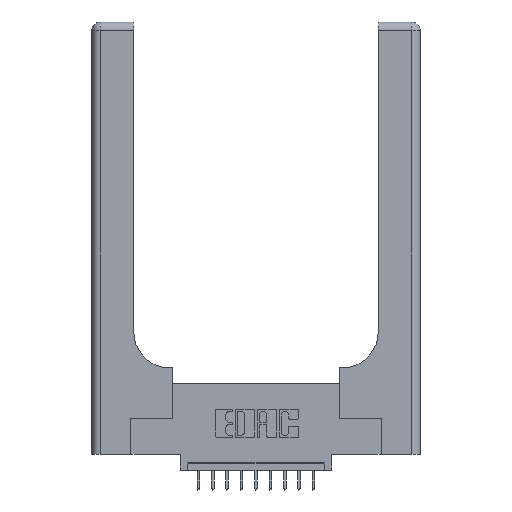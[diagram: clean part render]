
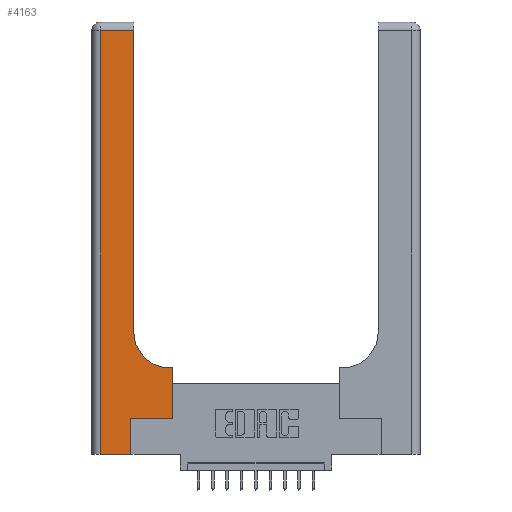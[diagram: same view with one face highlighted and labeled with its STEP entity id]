
A CAD part, top view. The second image highlights one B-rep face of the part: STEP entity #4163.
In plain terms, the highlighted planar face has unit normal (0, 0, 1).
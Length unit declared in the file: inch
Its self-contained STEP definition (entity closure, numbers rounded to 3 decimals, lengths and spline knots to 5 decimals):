
#88 = CARTESIAN_POINT ( 'NONE',  ( 0.5585, 0.6, 0.37 ) ) ;
#327 = VECTOR ( 'NONE', #10025, 39.37008 ) ;
#654 = ORIENTED_EDGE ( 'NONE', *, *, #2402, .T. ) ;
#759 = CARTESIAN_POINT ( 'NONE',  ( 0.5585, 0.25, 0.37 ) ) ;
#824 = CARTESIAN_POINT ( 'NONE',  ( 0.5415, 0.6, 0.37 ) ) ;
#992 = CARTESIAN_POINT ( 'NONE',  ( 0., 2.94, 0.37 ) ) ;
#1068 = VECTOR ( 'NONE', #10743, 39.37008 ) ;
#1175 = EDGE_CURVE ( 'NONE', #6383, #5302, #15178, .T. ) ;
#1339 = DIRECTION ( 'NONE',  ( 0., 1., 0. ) ) ;
#1602 = EDGE_LOOP ( 'NONE', ( #10691, #9504, #8121, #3384, #654, #14400, #3420, #8779, #9901 ) ) ;
#1735 = CARTESIAN_POINT ( 'NONE',  ( 0.269, 0., 0.37 ) ) ;
#2074 = EDGE_CURVE ( 'NONE', #12325, #16010, #11331, .T. ) ;
#2081 = CARTESIAN_POINT ( 'NONE',  ( 0.269, 0.25, 0.37 ) ) ;
#2402 = EDGE_CURVE ( 'NONE', #16010, #4941, #10570, .T. ) ;
#2519 = VECTOR ( 'NONE', #8267, 39.37008 ) ;
#2576 = EDGE_CURVE ( 'NONE', #12427, #7344, #16180, .T. ) ;
#3227 = CARTESIAN_POINT ( 'NONE',  ( 0.269, 0.25, 0.37 ) ) ;
#3384 = ORIENTED_EDGE ( 'NONE', *, *, #2074, .T. ) ;
#3420 = ORIENTED_EDGE ( 'NONE', *, *, #2576, .T. ) ;
#3853 = CARTESIAN_POINT ( 'NONE',  ( 0.06, 2.94, 0.37 ) ) ;
#4128 = EDGE_CURVE ( 'NONE', #7344, #5515, #15139, .T. ) ;
#4163 = ADVANCED_FACE ( 'NONE', ( #5919 ), #11055, .F. ) ;
#4760 = CARTESIAN_POINT ( 'NONE',  ( 0.06, 3., 0.37 ) ) ;
#4821 = CIRCLE ( 'NONE', #10686, 0.25 ) ;
#4869 = CARTESIAN_POINT ( 'NONE',  ( 0.5415, 0.85, 0.37 ) ) ;
#4941 = VERTEX_POINT ( 'NONE', #2081 ) ;
#5048 = CARTESIAN_POINT ( 'NONE',  ( 0., 0., 0.37 ) ) ;
#5246 = VECTOR ( 'NONE', #13818, 39.37008 ) ;
#5302 = VERTEX_POINT ( 'NONE', #8695 ) ;
#5343 = VECTOR ( 'NONE', #8303, 39.37008 ) ;
#5515 = VERTEX_POINT ( 'NONE', #824 ) ;
#5919 = FACE_OUTER_BOUND ( 'NONE', #1602, .T. ) ;
#6294 = VERTEX_POINT ( 'NONE', #3853 ) ;
#6383 = VERTEX_POINT ( 'NONE', #10905 ) ;
#7344 = VERTEX_POINT ( 'NONE', #88 ) ;
#7688 = CARTESIAN_POINT ( 'NONE',  ( 0.06, 0., 0.37 ) ) ;
#8121 = ORIENTED_EDGE ( 'NONE', *, *, #8969, .T. ) ;
#8267 = DIRECTION ( 'NONE',  ( 1., 0., 0. ) ) ;
#8303 = DIRECTION ( 'NONE',  ( 0., 1., 0. ) ) ;
#8522 = CARTESIAN_POINT ( 'NONE',  ( 0., 3., 0.37 ) ) ;
#8695 = CARTESIAN_POINT ( 'NONE',  ( 0.2915, 2.94, 0.37 ) ) ;
#8779 = ORIENTED_EDGE ( 'NONE', *, *, #4128, .T. ) ;
#8969 = EDGE_CURVE ( 'NONE', #6294, #12325, #12407, .T. ) ;
#9504 = ORIENTED_EDGE ( 'NONE', *, *, #11136, .T. ) ;
#9632 = EDGE_CURVE ( 'NONE', #4941, #12427, #14793, .T. ) ;
#9901 = ORIENTED_EDGE ( 'NONE', *, *, #12830, .T. ) ;
#10004 = VECTOR ( 'NONE', #11797, 39.37008 ) ;
#10025 = DIRECTION ( 'NONE',  ( -1., 0., 0. ) ) ;
#10426 = VECTOR ( 'NONE', #14485, 39.37008 ) ;
#10570 = LINE ( 'NONE', #1735, #1068 ) ;
#10686 = AXIS2_PLACEMENT_3D ( 'NONE', #4869, #11166, #13578 ) ;
#10691 = ORIENTED_EDGE ( 'NONE', *, *, #1175, .T. ) ;
#10743 = DIRECTION ( 'NONE',  ( 0., 1., 0. ) ) ;
#10905 = CARTESIAN_POINT ( 'NONE',  ( 0.2915, 0.85, 0.37 ) ) ;
#11055 = PLANE ( 'NONE',  #13509 ) ;
#11136 = EDGE_CURVE ( 'NONE', #5302, #6294, #16326, .T. ) ;
#11166 = DIRECTION ( 'NONE',  ( 0., 0., -1. ) ) ;
#11331 = LINE ( 'NONE', #5048, #10426 ) ;
#11797 = DIRECTION ( 'NONE',  ( 0., -1., 0. ) ) ;
#12325 = VERTEX_POINT ( 'NONE', #7688 ) ;
#12407 = LINE ( 'NONE', #4760, #10004 ) ;
#12426 = DIRECTION ( 'NONE',  ( 0., 0., -1. ) ) ;
#12427 = VERTEX_POINT ( 'NONE', #15809 ) ;
#12830 = EDGE_CURVE ( 'NONE', #5515, #6383, #4821, .T. ) ;
#13509 = AXIS2_PLACEMENT_3D ( 'NONE', #8522, #12426, #16314 ) ;
#13578 = DIRECTION ( 'NONE',  ( 1., 0., 0. ) ) ;
#13818 = DIRECTION ( 'NONE',  ( -1., 0., 0. ) ) ;
#14400 = ORIENTED_EDGE ( 'NONE', *, *, #9632, .T. ) ;
#14485 = DIRECTION ( 'NONE',  ( 1., 0., 0. ) ) ;
#14793 = LINE ( 'NONE', #3227, #2519 ) ;
#15139 = LINE ( 'NONE', #16237, #327 ) ;
#15178 = LINE ( 'NONE', #15346, #15353 ) ;
#15346 = CARTESIAN_POINT ( 'NONE',  ( 0.2915, 3., 0.37 ) ) ;
#15353 = VECTOR ( 'NONE', #1339, 39.37008 ) ;
#15409 = CARTESIAN_POINT ( 'NONE',  ( 0.269, 0., 0.37 ) ) ;
#15809 = CARTESIAN_POINT ( 'NONE',  ( 0.5585, 0.25, 0.37 ) ) ;
#16010 = VERTEX_POINT ( 'NONE', #15409 ) ;
#16180 = LINE ( 'NONE', #759, #5343 ) ;
#16237 = CARTESIAN_POINT ( 'NONE',  ( 0.2915, 0.6, 0.37 ) ) ;
#16314 = DIRECTION ( 'NONE',  ( -1., 0., 0. ) ) ;
#16326 = LINE ( 'NONE', #992, #5246 ) ;
